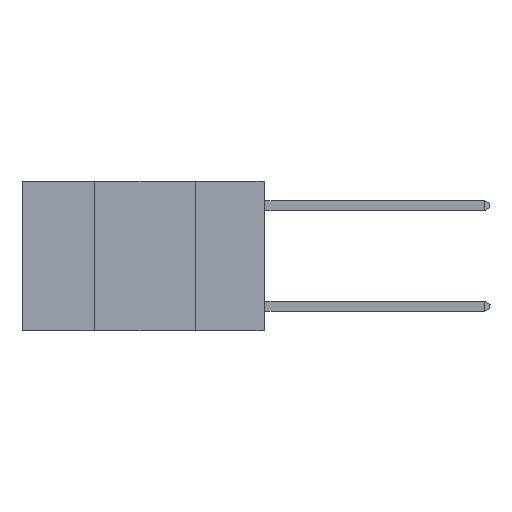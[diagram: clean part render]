
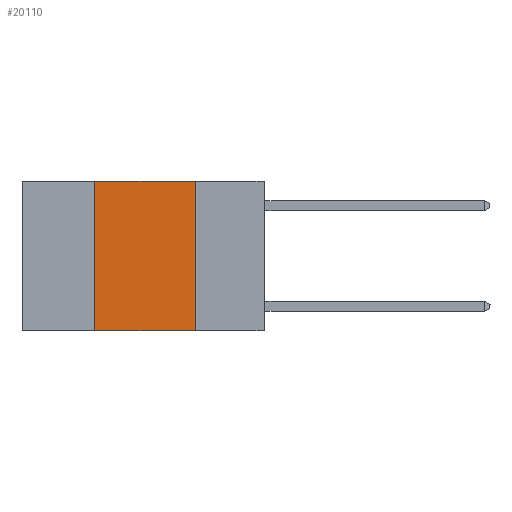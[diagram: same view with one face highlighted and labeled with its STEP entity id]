
A CAD part, left-side view. The second image highlights one B-rep face of the part: STEP entity #20110.
In plain terms, the highlighted planar face has unit normal (-1, 0, 0).
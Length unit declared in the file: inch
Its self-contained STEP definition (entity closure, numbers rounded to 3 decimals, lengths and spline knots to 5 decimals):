
#2844 = VECTOR ( 'NONE', #10010, 39.37008 ) ;
#2940 = VERTEX_POINT ( 'NONE', #9929 ) ;
#4091 = CARTESIAN_POINT ( 'NONE',  ( 0., 0.42, -0.37 ) ) ;
#4502 = VERTEX_POINT ( 'NONE', #4091 ) ;
#4510 = DIRECTION ( 'NONE',  ( 0., 0., 1. ) ) ;
#5249 = ORIENTED_EDGE ( 'NONE', *, *, #12933, .F. ) ;
#5542 = DIRECTION ( 'NONE',  ( 0., -1., 0. ) ) ;
#6015 = CARTESIAN_POINT ( 'NONE',  ( 0., 0.17, 0. ) ) ;
#6291 = EDGE_LOOP ( 'NONE', ( #25888, #5249, #27549, #26763 ) ) ;
#6559 = EDGE_CURVE ( 'NONE', #4502, #8576, #15797, .T. ) ;
#6949 = CARTESIAN_POINT ( 'NONE',  ( 0., 0.42, 0. ) ) ;
#7311 = DIRECTION ( 'NONE',  ( 0., 0., -1. ) ) ;
#8576 = VERTEX_POINT ( 'NONE', #6949 ) ;
#9502 = VECTOR ( 'NONE', #4510, 39.37008 ) ;
#9929 = CARTESIAN_POINT ( 'NONE',  ( 0., 0.17, -0.37 ) ) ;
#10010 = DIRECTION ( 'NONE',  ( 0., -1., 0. ) ) ;
#10539 = LINE ( 'NONE', #28976, #23199 ) ;
#12611 = CARTESIAN_POINT ( 'NONE',  ( 0., 0.6, 0. ) ) ;
#12933 = EDGE_CURVE ( 'NONE', #8576, #20429, #18084, .T. ) ;
#14349 = CARTESIAN_POINT ( 'NONE',  ( 0., 0.6, 0. ) ) ;
#14692 = DIRECTION ( 'NONE',  ( 0., 0., -1. ) ) ;
#14735 = LINE ( 'NONE', #26665, #2844 ) ;
#15797 = LINE ( 'NONE', #21185, #9502 ) ;
#18084 = LINE ( 'NONE', #12611, #30002 ) ;
#19158 = PLANE ( 'NONE',  #25020 ) ;
#20110 = ADVANCED_FACE ( 'NONE', ( #25532 ), #19158, .F. ) ;
#20429 = VERTEX_POINT ( 'NONE', #6015 ) ;
#21185 = CARTESIAN_POINT ( 'NONE',  ( 0., 0.42, 0. ) ) ;
#21548 = EDGE_CURVE ( 'NONE', #20429, #2940, #10539, .T. ) ;
#21580 = DIRECTION ( 'NONE',  ( 1., 0., 0. ) ) ;
#23199 = VECTOR ( 'NONE', #14692, 39.37008 ) ;
#25020 = AXIS2_PLACEMENT_3D ( 'NONE', #14349, #21580, #7311 ) ;
#25532 = FACE_OUTER_BOUND ( 'NONE', #6291, .T. ) ;
#25888 = ORIENTED_EDGE ( 'NONE', *, *, #21548, .F. ) ;
#26665 = CARTESIAN_POINT ( 'NONE',  ( 0., 0.6, -0.37 ) ) ;
#26763 = ORIENTED_EDGE ( 'NONE', *, *, #27308, .T. ) ;
#27308 = EDGE_CURVE ( 'NONE', #4502, #2940, #14735, .T. ) ;
#27549 = ORIENTED_EDGE ( 'NONE', *, *, #6559, .F. ) ;
#28976 = CARTESIAN_POINT ( 'NONE',  ( 0., 0.17, 0. ) ) ;
#30002 = VECTOR ( 'NONE', #5542, 39.37008 ) ;
